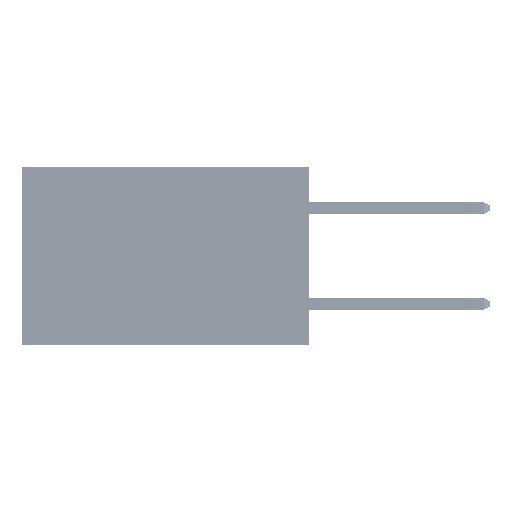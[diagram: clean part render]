
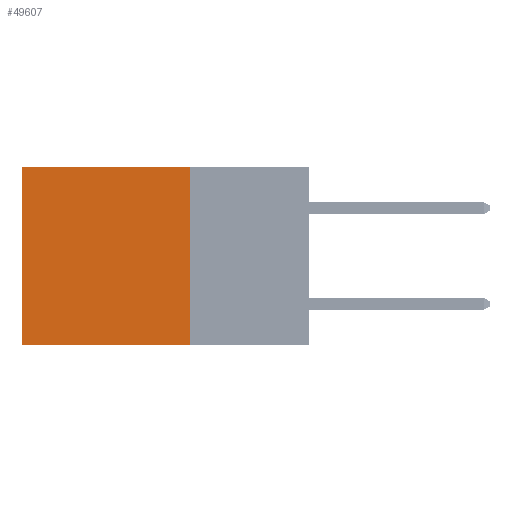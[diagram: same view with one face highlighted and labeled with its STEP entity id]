
A CAD part, left-side view. The second image highlights one B-rep face of the part: STEP entity #49607.
In plain terms, the highlighted planar face has unit normal (-1, 0, 0).
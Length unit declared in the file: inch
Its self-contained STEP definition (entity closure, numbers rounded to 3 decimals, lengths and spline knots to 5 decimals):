
#1634 = CARTESIAN_POINT ( 'NONE',  ( 0.2875, 0.6, 0. ) ) ;
#3090 = EDGE_LOOP ( 'NONE', ( #37840, #40041, #13847, #18526 ) ) ;
#9170 = DIRECTION ( 'NONE',  ( 0., 1., 0. ) ) ;
#9689 = DIRECTION ( 'NONE',  ( 0., 0., -1. ) ) ;
#9913 = CARTESIAN_POINT ( 'NONE',  ( 0.2875, 0.25, -0.37 ) ) ;
#13726 = LINE ( 'NONE', #28321, #46203 ) ;
#13847 = ORIENTED_EDGE ( 'NONE', *, *, #49127, .F. ) ;
#14298 = FACE_OUTER_BOUND ( 'NONE', #3090, .T. ) ;
#15179 = VERTEX_POINT ( 'NONE', #25759 ) ;
#18322 = PLANE ( 'NONE',  #38237 ) ;
#18526 = ORIENTED_EDGE ( 'NONE', *, *, #24967, .T. ) ;
#18565 = DIRECTION ( 'NONE',  ( 1., 0., 0. ) ) ;
#19505 = EDGE_CURVE ( 'NONE', #21637, #15179, #36318, .T. ) ;
#21542 = VECTOR ( 'NONE', #9689, 39.37008 ) ;
#21637 = VERTEX_POINT ( 'NONE', #30974 ) ;
#21727 = CARTESIAN_POINT ( 'NONE',  ( 0.2875, 0.25, 0. ) ) ;
#23664 = EDGE_CURVE ( 'NONE', #24799, #15179, #43859, .T. ) ;
#24799 = VERTEX_POINT ( 'NONE', #34400 ) ;
#24967 = EDGE_CURVE ( 'NONE', #27707, #21637, #28792, .T. ) ;
#25759 = CARTESIAN_POINT ( 'NONE',  ( 0.2875, 0.6, -0.37 ) ) ;
#27707 = VERTEX_POINT ( 'NONE', #48879 ) ;
#28321 = CARTESIAN_POINT ( 'NONE',  ( 0.2875, 0.25, 0. ) ) ;
#28792 = LINE ( 'NONE', #21727, #42420 ) ;
#30974 = CARTESIAN_POINT ( 'NONE',  ( 0.2875, 0.6, 0. ) ) ;
#31485 = VECTOR ( 'NONE', #9170, 39.37008 ) ;
#31842 = DIRECTION ( 'NONE',  ( 0., 0., -1. ) ) ;
#34400 = CARTESIAN_POINT ( 'NONE',  ( 0.2875, 0.25, -0.37 ) ) ;
#36318 = LINE ( 'NONE', #1634, #21542 ) ;
#37840 = ORIENTED_EDGE ( 'NONE', *, *, #19505, .T. ) ;
#38237 = AXIS2_PLACEMENT_3D ( 'NONE', #41457, #18565, #47385 ) ;
#40041 = ORIENTED_EDGE ( 'NONE', *, *, #23664, .F. ) ;
#41457 = CARTESIAN_POINT ( 'NONE',  ( 0.2875, 0.25, 0. ) ) ;
#42420 = VECTOR ( 'NONE', #43866, 39.37008 ) ;
#43859 = LINE ( 'NONE', #9913, #31485 ) ;
#43866 = DIRECTION ( 'NONE',  ( 0., 1., 0. ) ) ;
#46203 = VECTOR ( 'NONE', #31842, 39.37008 ) ;
#47385 = DIRECTION ( 'NONE',  ( 0., 0., -1. ) ) ;
#48879 = CARTESIAN_POINT ( 'NONE',  ( 0.2875, 0.25, 0. ) ) ;
#49127 = EDGE_CURVE ( 'NONE', #27707, #24799, #13726, .T. ) ;
#49607 = ADVANCED_FACE ( 'NONE', ( #14298 ), #18322, .F. ) ;
